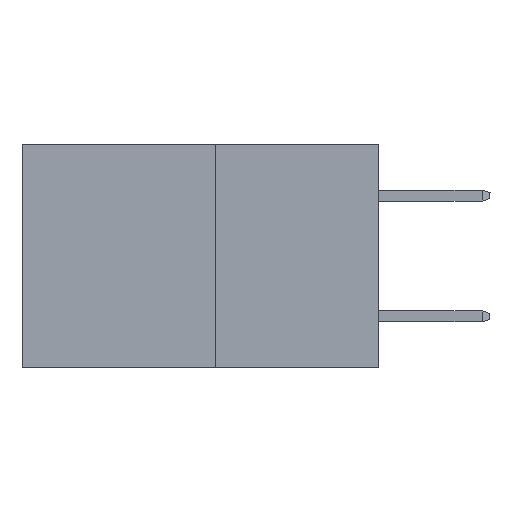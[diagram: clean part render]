
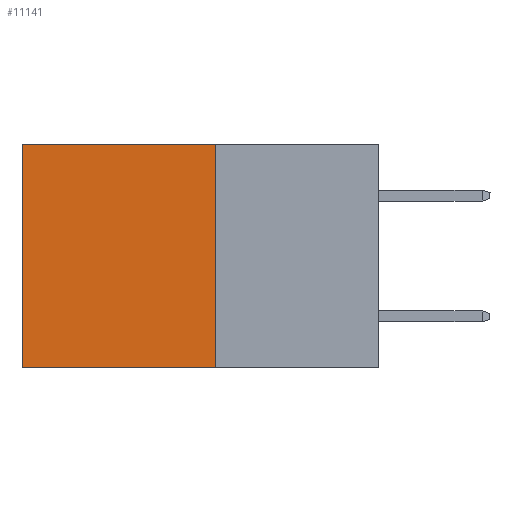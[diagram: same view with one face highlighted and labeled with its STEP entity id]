
A CAD part, left-side view. The second image highlights one B-rep face of the part: STEP entity #11141.
In plain terms, the highlighted planar face has unit normal (-1, 0, 0).
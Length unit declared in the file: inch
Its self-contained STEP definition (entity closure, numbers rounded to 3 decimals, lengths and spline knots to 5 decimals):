
#64 = VECTOR ( 'NONE', #10622, 39.37008 ) ;
#1200 = DIRECTION ( 'NONE',  ( 0., 0., -1. ) ) ;
#1585 = CARTESIAN_POINT ( 'NONE',  ( 0.277, 0.59, -0.37 ) ) ;
#1974 = EDGE_CURVE ( 'NONE', #7104, #3606, #10206, .T. ) ;
#2087 = FACE_OUTER_BOUND ( 'NONE', #5872, .T. ) ;
#2429 = VECTOR ( 'NONE', #1200, 39.37008 ) ;
#2456 = CARTESIAN_POINT ( 'NONE',  ( 0.277, 0.27, -0.37 ) ) ;
#2839 = ORIENTED_EDGE ( 'NONE', *, *, #8073, .F. ) ;
#2884 = CARTESIAN_POINT ( 'NONE',  ( 0.277, 0.27, 0. ) ) ;
#3309 = CARTESIAN_POINT ( 'NONE',  ( 0.277, 0.27, -0.37 ) ) ;
#3606 = VERTEX_POINT ( 'NONE', #7982 ) ;
#3645 = CARTESIAN_POINT ( 'NONE',  ( 0.277, 0.27, -0.37 ) ) ;
#4442 = EDGE_CURVE ( 'NONE', #7104, #6958, #5640, .T. ) ;
#4537 = CARTESIAN_POINT ( 'NONE',  ( 0.277, 0.27, -0.37 ) ) ;
#4833 = DIRECTION ( 'NONE',  ( 0., 0., -1. ) ) ;
#4900 = VECTOR ( 'NONE', #7510, 39.37008 ) ;
#5556 = VECTOR ( 'NONE', #4833, 39.37008 ) ;
#5640 = LINE ( 'NONE', #3309, #2429 ) ;
#5872 = EDGE_LOOP ( 'NONE', ( #8195, #2839, #8521, #12994 ) ) ;
#6878 = DIRECTION ( 'NONE',  ( 0., 0., -1. ) ) ;
#6958 = VERTEX_POINT ( 'NONE', #3645 ) ;
#7104 = VERTEX_POINT ( 'NONE', #12351 ) ;
#7201 = VERTEX_POINT ( 'NONE', #10372 ) ;
#7510 = DIRECTION ( 'NONE',  ( 0., 1., 0. ) ) ;
#7825 = AXIS2_PLACEMENT_3D ( 'NONE', #4537, #9831, #6878 ) ;
#7982 = CARTESIAN_POINT ( 'NONE',  ( 0.277, 0.59, 0. ) ) ;
#8073 = EDGE_CURVE ( 'NONE', #6958, #7201, #11035, .T. ) ;
#8195 = ORIENTED_EDGE ( 'NONE', *, *, #8292, .T. ) ;
#8292 = EDGE_CURVE ( 'NONE', #3606, #7201, #8734, .T. ) ;
#8521 = ORIENTED_EDGE ( 'NONE', *, *, #4442, .F. ) ;
#8734 = LINE ( 'NONE', #1585, #5556 ) ;
#9831 = DIRECTION ( 'NONE',  ( 1., 0., 0. ) ) ;
#10206 = LINE ( 'NONE', #2884, #4900 ) ;
#10372 = CARTESIAN_POINT ( 'NONE',  ( 0.277, 0.59, -0.37 ) ) ;
#10622 = DIRECTION ( 'NONE',  ( 0., 1., 0. ) ) ;
#11035 = LINE ( 'NONE', #2456, #64 ) ;
#11141 = ADVANCED_FACE ( 'NONE', ( #2087 ), #13045, .F. ) ;
#12351 = CARTESIAN_POINT ( 'NONE',  ( 0.277, 0.27, 0. ) ) ;
#12994 = ORIENTED_EDGE ( 'NONE', *, *, #1974, .T. ) ;
#13045 = PLANE ( 'NONE',  #7825 ) ;
